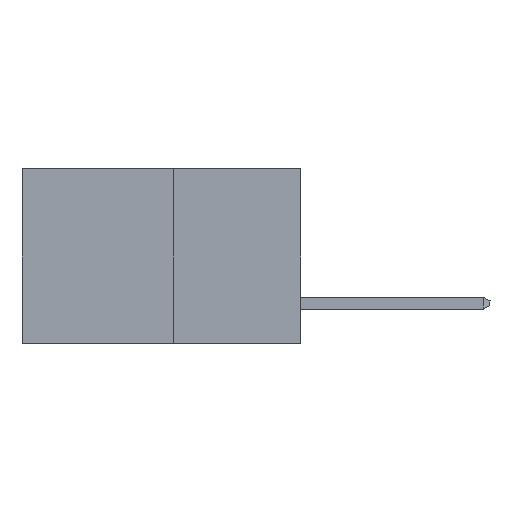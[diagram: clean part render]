
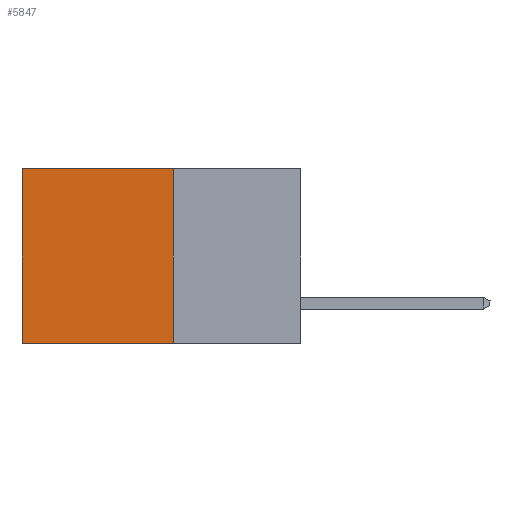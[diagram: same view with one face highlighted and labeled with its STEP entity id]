
A CAD part, left-side view. The second image highlights one B-rep face of the part: STEP entity #5847.
In plain terms, the highlighted planar face has unit normal (-1, 0, 0).
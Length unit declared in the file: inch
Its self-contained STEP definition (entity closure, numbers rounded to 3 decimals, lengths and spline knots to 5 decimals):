
#225 = VERTEX_POINT ( 'NONE', #1960 ) ;
#755 = EDGE_CURVE ( 'NONE', #2534, #4661, #3802, .T. ) ;
#790 = EDGE_CURVE ( 'NONE', #225, #2534, #8576, .T. ) ;
#1028 = AXIS2_PLACEMENT_3D ( 'NONE', #7225, #7124, #7112 ) ;
#1280 = ORIENTED_EDGE ( 'NONE', *, *, #1994, .T. ) ;
#1405 = DIRECTION ( 'NONE',  ( 0., 1., 0. ) ) ;
#1470 = LINE ( 'NONE', #3655, #7180 ) ;
#1960 = CARTESIAN_POINT ( 'NONE',  ( 0.277, 0.27, 0. ) ) ;
#1994 = EDGE_CURVE ( 'NONE', #7459, #4661, #3317, .T. ) ;
#2534 = VERTEX_POINT ( 'NONE', #5425 ) ;
#2821 = VECTOR ( 'NONE', #7816, 39.37008 ) ;
#2855 = ORIENTED_EDGE ( 'NONE', *, *, #755, .F. ) ;
#3317 = LINE ( 'NONE', #9248, #8794 ) ;
#3387 = EDGE_CURVE ( 'NONE', #225, #7459, #1470, .T. ) ;
#3655 = CARTESIAN_POINT ( 'NONE',  ( 0.277, 0.27, 0. ) ) ;
#3697 = ORIENTED_EDGE ( 'NONE', *, *, #3387, .T. ) ;
#3729 = DIRECTION ( 'NONE',  ( 0., 1., 0. ) ) ;
#3802 = LINE ( 'NONE', #4512, #8801 ) ;
#4241 = CARTESIAN_POINT ( 'NONE',  ( 0.277, 0.59, -0.37 ) ) ;
#4317 = FACE_OUTER_BOUND ( 'NONE', #4893, .T. ) ;
#4512 = CARTESIAN_POINT ( 'NONE',  ( 0.277, 0.27, -0.37 ) ) ;
#4661 = VERTEX_POINT ( 'NONE', #4241 ) ;
#4868 = CARTESIAN_POINT ( 'NONE',  ( 0.277, 0.27, -0.37 ) ) ;
#4893 = EDGE_LOOP ( 'NONE', ( #1280, #2855, #7917, #3697 ) ) ;
#5425 = CARTESIAN_POINT ( 'NONE',  ( 0.277, 0.27, -0.37 ) ) ;
#5847 = ADVANCED_FACE ( 'NONE', ( #4317 ), #7254, .F. ) ;
#7112 = DIRECTION ( 'NONE',  ( 0., 0., -1. ) ) ;
#7124 = DIRECTION ( 'NONE',  ( 1., 0., 0. ) ) ;
#7180 = VECTOR ( 'NONE', #3729, 39.37008 ) ;
#7225 = CARTESIAN_POINT ( 'NONE',  ( 0.277, 0.27, -0.37 ) ) ;
#7254 = PLANE ( 'NONE',  #1028 ) ;
#7459 = VERTEX_POINT ( 'NONE', #7724 ) ;
#7724 = CARTESIAN_POINT ( 'NONE',  ( 0.277, 0.59, 0. ) ) ;
#7816 = DIRECTION ( 'NONE',  ( 0., 0., -1. ) ) ;
#7917 = ORIENTED_EDGE ( 'NONE', *, *, #790, .F. ) ;
#7977 = DIRECTION ( 'NONE',  ( 0., 0., -1. ) ) ;
#8576 = LINE ( 'NONE', #4868, #2821 ) ;
#8794 = VECTOR ( 'NONE', #7977, 39.37008 ) ;
#8801 = VECTOR ( 'NONE', #1405, 39.37008 ) ;
#9248 = CARTESIAN_POINT ( 'NONE',  ( 0.277, 0.59, -0.37 ) ) ;
